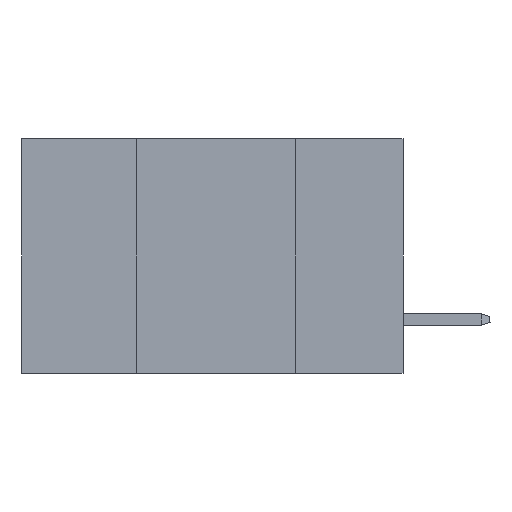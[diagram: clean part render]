
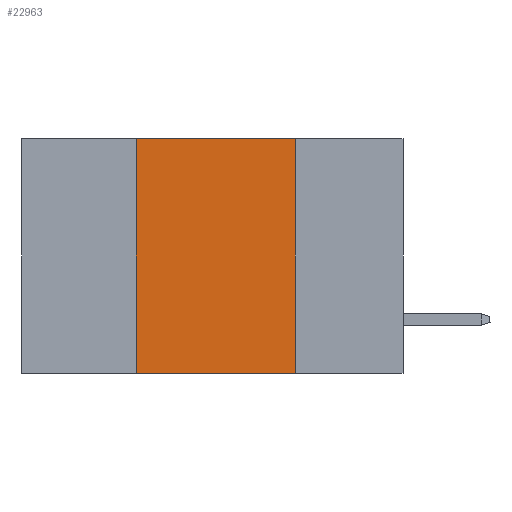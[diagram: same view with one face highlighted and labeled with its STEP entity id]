
A CAD part, left-side view. The second image highlights one B-rep face of the part: STEP entity #22963.
In plain terms, the highlighted planar face has unit normal (-1, 0, 0).
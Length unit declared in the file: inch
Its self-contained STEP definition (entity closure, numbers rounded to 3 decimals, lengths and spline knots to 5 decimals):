
#2035 = LINE ( 'NONE', #26497, #11618 ) ;
#2623 = LINE ( 'NONE', #30829, #45673 ) ;
#2767 = AXIS2_PLACEMENT_3D ( 'NONE', #24371, #20629, #9913 ) ;
#3910 = ORIENTED_EDGE ( 'NONE', *, *, #32677, .F. ) ;
#7200 = DIRECTION ( 'NONE',  ( 0., 0., -1. ) ) ;
#8044 = EDGE_LOOP ( 'NONE', ( #26318, #12855, #3910, #34481 ) ) ;
#8282 = DIRECTION ( 'NONE',  ( 0., -1., 0. ) ) ;
#9913 = DIRECTION ( 'NONE',  ( 0., 0., -1. ) ) ;
#10340 = DIRECTION ( 'NONE',  ( 0., -1., 0. ) ) ;
#11618 = VECTOR ( 'NONE', #12968, 39.37008 ) ;
#12855 = ORIENTED_EDGE ( 'NONE', *, *, #32452, .F. ) ;
#12968 = DIRECTION ( 'NONE',  ( 0., 0., 1. ) ) ;
#17727 = CARTESIAN_POINT ( 'NONE',  ( 0., 0.17, -0.37 ) ) ;
#18545 = CARTESIAN_POINT ( 'NONE',  ( 0., 0.42, -0.37 ) ) ;
#20629 = DIRECTION ( 'NONE',  ( 1., 0., 0. ) ) ;
#21366 = VERTEX_POINT ( 'NONE', #28593 ) ;
#22963 = ADVANCED_FACE ( 'NONE', ( #44153 ), #28325, .F. ) ;
#24371 = CARTESIAN_POINT ( 'NONE',  ( 0., 0.6, 0. ) ) ;
#24453 = VECTOR ( 'NONE', #8282, 39.37008 ) ;
#24729 = CARTESIAN_POINT ( 'NONE',  ( 0., 0.42, 0. ) ) ;
#25236 = CARTESIAN_POINT ( 'NONE',  ( 0., 0.6, 0. ) ) ;
#26318 = ORIENTED_EDGE ( 'NONE', *, *, #43039, .F. ) ;
#26497 = CARTESIAN_POINT ( 'NONE',  ( 0., 0.42, 0. ) ) ;
#27995 = VECTOR ( 'NONE', #10340, 39.37008 ) ;
#28325 = PLANE ( 'NONE',  #2767 ) ;
#28593 = CARTESIAN_POINT ( 'NONE',  ( 0., 0.17, 0. ) ) ;
#30829 = CARTESIAN_POINT ( 'NONE',  ( 0., 0.17, 0. ) ) ;
#32452 = EDGE_CURVE ( 'NONE', #32926, #21366, #38763, .T. ) ;
#32677 = EDGE_CURVE ( 'NONE', #35230, #32926, #2035, .T. ) ;
#32926 = VERTEX_POINT ( 'NONE', #24729 ) ;
#34481 = ORIENTED_EDGE ( 'NONE', *, *, #35273, .T. ) ;
#35230 = VERTEX_POINT ( 'NONE', #18545 ) ;
#35273 = EDGE_CURVE ( 'NONE', #35230, #40041, #40195, .T. ) ;
#38763 = LINE ( 'NONE', #25236, #27995 ) ;
#40041 = VERTEX_POINT ( 'NONE', #17727 ) ;
#40195 = LINE ( 'NONE', #43220, #24453 ) ;
#43039 = EDGE_CURVE ( 'NONE', #21366, #40041, #2623, .T. ) ;
#43220 = CARTESIAN_POINT ( 'NONE',  ( 0., 0.6, -0.37 ) ) ;
#44153 = FACE_OUTER_BOUND ( 'NONE', #8044, .T. ) ;
#45673 = VECTOR ( 'NONE', #7200, 39.37008 ) ;
